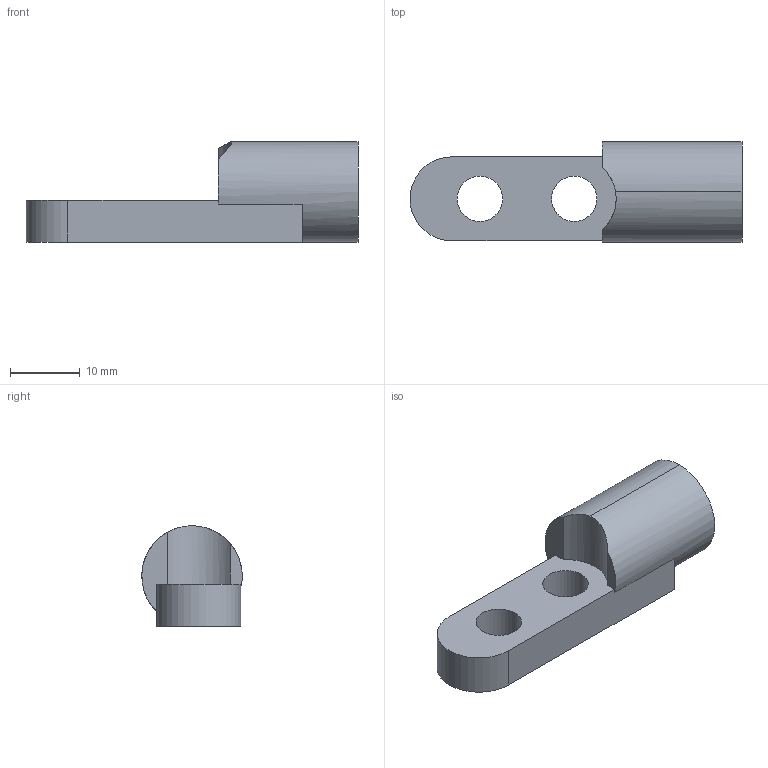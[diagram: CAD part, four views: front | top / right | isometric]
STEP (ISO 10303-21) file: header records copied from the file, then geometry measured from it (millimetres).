
FILE_DESCRIPTION (( 'STEP AP203' ), '1' );
FILE_NAME ('BufferToFCG_Left.STEP', '2019-09-03T07:07:02', ( '' ), ( '' ), 'SwSTEP 2.0', 'SolidWorks 2018', '' );
FILE_SCHEMA (( 'CONFIG_CONTROL_DESIGN' ));
Length unit declared in the file: millimetre
Products named in the file (1): BufferToFCG_Left
Bounding box: 47.5 x 14.36 x 14.36 mm (x, y, z)
Volume: 4402.4 mm3; surface area: 2603.8 mm2
Topology: 1 solids, 1 shells, 21 faces, 55 edges, 35 vertices
Faces by surface type: cylinder 10, plane 9, sphere 2
Entity records: 731 total; most frequent: CARTESIAN_POINT 132, DIRECTION 116, ORIENTED_EDGE 102, EDGE_CURVE 51, AXIS2_PLACEMENT_3D 45, VERTEX_POINT 33, EDGE_LOOP 26, LINE 26
